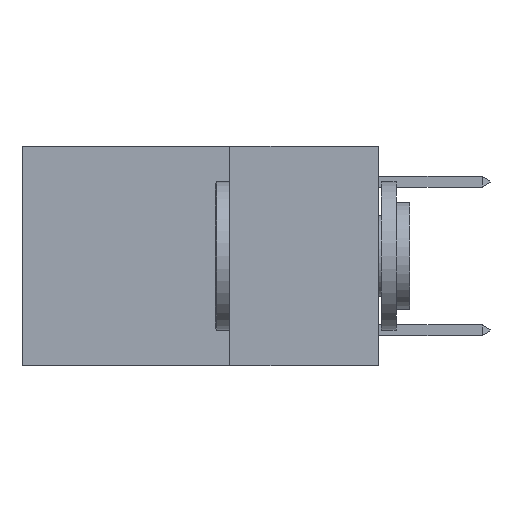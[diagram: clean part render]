
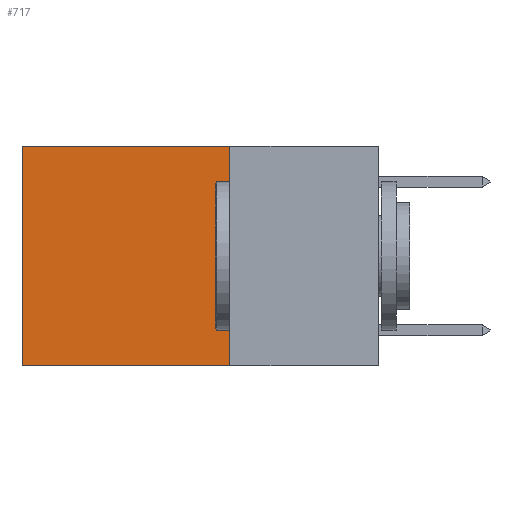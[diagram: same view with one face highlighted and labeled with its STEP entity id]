
A CAD part, left-side view. The second image highlights one B-rep face of the part: STEP entity #717.
In plain terms, the highlighted planar face has unit normal (-1, 0, 0).
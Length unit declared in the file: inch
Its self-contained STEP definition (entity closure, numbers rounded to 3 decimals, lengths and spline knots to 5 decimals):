
#21 = AXIS2_PLACEMENT_3D ( 'NONE', #4862, #10296, #10049 ) ;
#697 = CARTESIAN_POINT ( 'NONE',  ( 0.2625, 0.25, 0. ) ) ;
#717 = ADVANCED_FACE ( 'NONE', ( #16554 ), #3587, .F. ) ;
#1424 = ORIENTED_EDGE ( 'NONE', *, *, #16183, .T. ) ;
#1543 = VECTOR ( 'NONE', #5993, 39.37008 ) ;
#1881 = EDGE_LOOP ( 'NONE', ( #1424, #3207, #10228, #14246 ) ) ;
#3158 = VERTEX_POINT ( 'NONE', #11415 ) ;
#3207 = ORIENTED_EDGE ( 'NONE', *, *, #5136, .F. ) ;
#3213 = LINE ( 'NONE', #11002, #1543 ) ;
#3409 = LINE ( 'NONE', #14878, #16662 ) ;
#3412 = VECTOR ( 'NONE', #11106, 39.37008 ) ;
#3587 = PLANE ( 'NONE',  #21 ) ;
#4862 = CARTESIAN_POINT ( 'NONE',  ( 0.2625, 0.25, 0. ) ) ;
#4936 = CARTESIAN_POINT ( 'NONE',  ( 0.2625, 0.25, -0.37 ) ) ;
#5136 = EDGE_CURVE ( 'NONE', #7901, #3158, #5446, .T. ) ;
#5286 = EDGE_CURVE ( 'NONE', #15030, #7191, #3409, .T. ) ;
#5446 = LINE ( 'NONE', #10636, #12358 ) ;
#5545 = CARTESIAN_POINT ( 'NONE',  ( 0.2625, 0.6, 0. ) ) ;
#5674 = LINE ( 'NONE', #14938, #3412 ) ;
#5993 = DIRECTION ( 'NONE',  ( 0., 0., -1. ) ) ;
#7191 = VERTEX_POINT ( 'NONE', #5545 ) ;
#7901 = VERTEX_POINT ( 'NONE', #4936 ) ;
#10049 = DIRECTION ( 'NONE',  ( 0., 0., -1. ) ) ;
#10228 = ORIENTED_EDGE ( 'NONE', *, *, #16615, .F. ) ;
#10296 = DIRECTION ( 'NONE',  ( 1., 0., 0. ) ) ;
#10636 = CARTESIAN_POINT ( 'NONE',  ( 0.2625, 0.25, -0.37 ) ) ;
#10801 = DIRECTION ( 'NONE',  ( 0., 1., 0. ) ) ;
#11002 = CARTESIAN_POINT ( 'NONE',  ( 0.2625, 0.25, 0. ) ) ;
#11106 = DIRECTION ( 'NONE',  ( 0., 0., -1. ) ) ;
#11415 = CARTESIAN_POINT ( 'NONE',  ( 0.2625, 0.6, -0.37 ) ) ;
#12358 = VECTOR ( 'NONE', #15803, 39.37008 ) ;
#14246 = ORIENTED_EDGE ( 'NONE', *, *, #5286, .T. ) ;
#14878 = CARTESIAN_POINT ( 'NONE',  ( 0.2625, 0.25, 0. ) ) ;
#14938 = CARTESIAN_POINT ( 'NONE',  ( 0.2625, 0.6, 0. ) ) ;
#15030 = VERTEX_POINT ( 'NONE', #697 ) ;
#15803 = DIRECTION ( 'NONE',  ( 0., 1., 0. ) ) ;
#16183 = EDGE_CURVE ( 'NONE', #7191, #3158, #5674, .T. ) ;
#16554 = FACE_OUTER_BOUND ( 'NONE', #1881, .T. ) ;
#16615 = EDGE_CURVE ( 'NONE', #15030, #7901, #3213, .T. ) ;
#16662 = VECTOR ( 'NONE', #10801, 39.37008 ) ;
